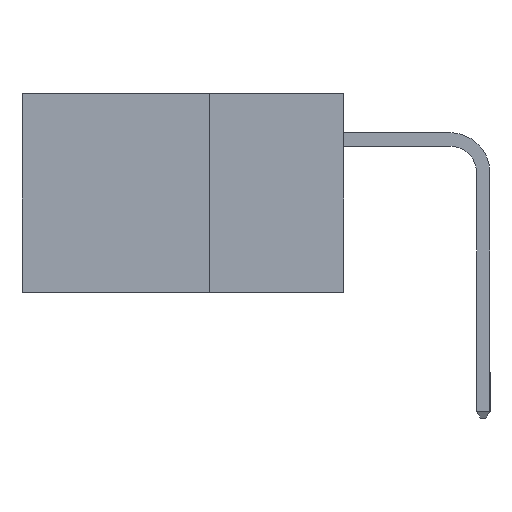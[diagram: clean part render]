
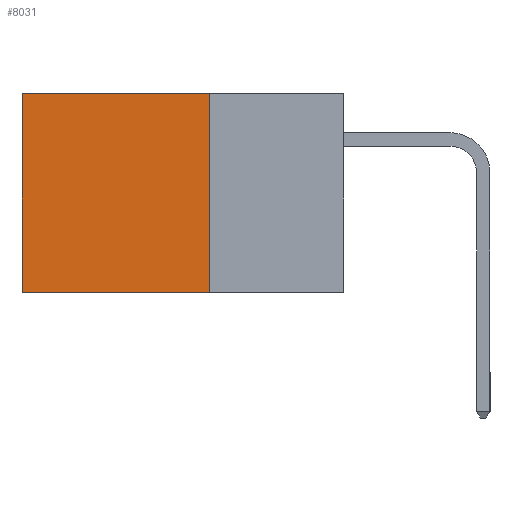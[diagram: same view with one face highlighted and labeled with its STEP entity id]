
A CAD part, left-side view. The second image highlights one B-rep face of the part: STEP entity #8031.
In plain terms, the highlighted planar face has unit normal (-1, 0, 0).
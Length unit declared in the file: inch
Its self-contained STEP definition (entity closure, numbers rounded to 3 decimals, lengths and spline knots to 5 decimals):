
#1146 = DIRECTION ( 'NONE',  ( 0., 0., -1. ) ) ;
#1169 = LINE ( 'NONE', #16522, #13582 ) ;
#1221 = EDGE_CURVE ( 'NONE', #10134, #16829, #2444, .T. ) ;
#2244 = ORIENTED_EDGE ( 'NONE', *, *, #1221, .F. ) ;
#2444 = LINE ( 'NONE', #2663, #16131 ) ;
#2663 = CARTESIAN_POINT ( 'NONE',  ( 0.298, 0.25, -0.37 ) ) ;
#2821 = DIRECTION ( 'NONE',  ( 0., 0., -1. ) ) ;
#3451 = ORIENTED_EDGE ( 'NONE', *, *, #15560, .T. ) ;
#3774 = EDGE_CURVE ( 'NONE', #5372, #10134, #16985, .T. ) ;
#3799 = VECTOR ( 'NONE', #7940, 39.37008 ) ;
#4450 = AXIS2_PLACEMENT_3D ( 'NONE', #14386, #12938, #1146 ) ;
#4645 = LINE ( 'NONE', #9070, #3799 ) ;
#4817 = EDGE_LOOP ( 'NONE', ( #3451, #2244, #9463, #15395 ) ) ;
#5351 = CARTESIAN_POINT ( 'NONE',  ( 0.298, 0.6, -0.37 ) ) ;
#5372 = VERTEX_POINT ( 'NONE', #16169 ) ;
#5993 = VECTOR ( 'NONE', #2821, 39.37008 ) ;
#6085 = DIRECTION ( 'NONE',  ( 0., 0., -1. ) ) ;
#6220 = DIRECTION ( 'NONE',  ( 0., 1., 0. ) ) ;
#7795 = CARTESIAN_POINT ( 'NONE',  ( 0.298, 0.25, -0.37 ) ) ;
#7940 = DIRECTION ( 'NONE',  ( 0., 1., 0. ) ) ;
#8031 = ADVANCED_FACE ( 'NONE', ( #16803 ), #15629, .F. ) ;
#8902 = CARTESIAN_POINT ( 'NONE',  ( 0.298, 0.6, 0. ) ) ;
#9070 = CARTESIAN_POINT ( 'NONE',  ( 0.298, 0.25, 0. ) ) ;
#9463 = ORIENTED_EDGE ( 'NONE', *, *, #3774, .F. ) ;
#10134 = VERTEX_POINT ( 'NONE', #7795 ) ;
#11512 = VERTEX_POINT ( 'NONE', #8902 ) ;
#12938 = DIRECTION ( 'NONE',  ( 1., 0., 0. ) ) ;
#13388 = CARTESIAN_POINT ( 'NONE',  ( 0.298, 0.25, 0. ) ) ;
#13582 = VECTOR ( 'NONE', #6085, 39.37008 ) ;
#14386 = CARTESIAN_POINT ( 'NONE',  ( 0.298, 0.25, 0. ) ) ;
#15395 = ORIENTED_EDGE ( 'NONE', *, *, #16825, .T. ) ;
#15560 = EDGE_CURVE ( 'NONE', #11512, #16829, #1169, .T. ) ;
#15629 = PLANE ( 'NONE',  #4450 ) ;
#16131 = VECTOR ( 'NONE', #6220, 39.37008 ) ;
#16169 = CARTESIAN_POINT ( 'NONE',  ( 0.298, 0.25, 0. ) ) ;
#16522 = CARTESIAN_POINT ( 'NONE',  ( 0.298, 0.6, 0. ) ) ;
#16803 = FACE_OUTER_BOUND ( 'NONE', #4817, .T. ) ;
#16825 = EDGE_CURVE ( 'NONE', #5372, #11512, #4645, .T. ) ;
#16829 = VERTEX_POINT ( 'NONE', #5351 ) ;
#16985 = LINE ( 'NONE', #13388, #5993 ) ;
